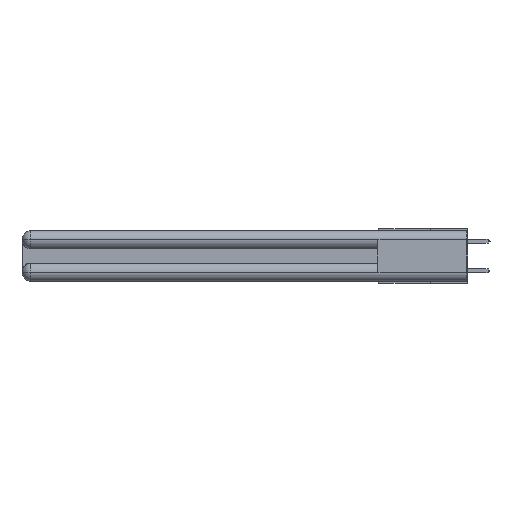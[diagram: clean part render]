
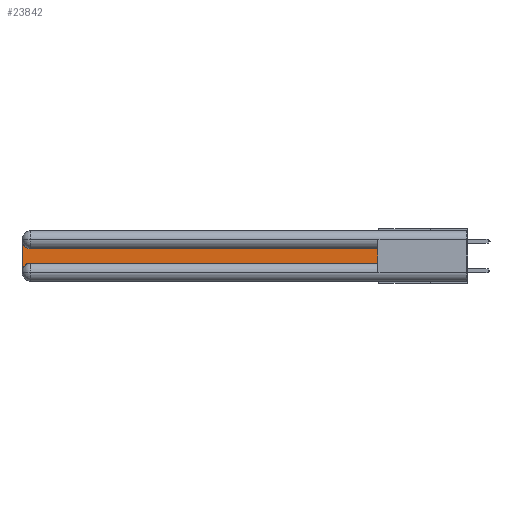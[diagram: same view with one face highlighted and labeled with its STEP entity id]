
A CAD part, left-side view. The second image highlights one B-rep face of the part: STEP entity #23842.
In plain terms, the highlighted planar face has unit normal (-1, 0, 0).
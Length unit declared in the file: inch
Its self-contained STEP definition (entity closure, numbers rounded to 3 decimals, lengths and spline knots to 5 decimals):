
#842 = VECTOR ( 'NONE', #8367, 39.37008 ) ;
#1450 = DIRECTION ( 'NONE',  ( 0., 0., -1. ) ) ;
#1662 = LINE ( 'NONE', #5142, #842 ) ;
#2708 = CARTESIAN_POINT ( 'NONE',  ( 0.075, 2.94, -0.0625 ) ) ;
#3270 = EDGE_LOOP ( 'NONE', ( #16878, #24091, #18093, #30044, #33054, #24185 ) ) ;
#4112 = LINE ( 'NONE', #25496, #29619 ) ;
#4541 = EDGE_CURVE ( 'NONE', #10692, #20927, #1662, .T. ) ;
#4879 = DIRECTION ( 'NONE',  ( 0., 0., -1. ) ) ;
#5142 = CARTESIAN_POINT ( 'NONE',  ( 0.075, 0.6, -0.2175 ) ) ;
#5673 = CIRCLE ( 'NONE', #33598, 0.06 ) ;
#5762 = VERTEX_POINT ( 'NONE', #7561 ) ;
#6572 = CARTESIAN_POINT ( 'NONE',  ( 0.075, 3., -0.0625 ) ) ;
#7421 = VECTOR ( 'NONE', #13288, 39.37008 ) ;
#7478 = EDGE_CURVE ( 'NONE', #5762, #22358, #5673, .T. ) ;
#7561 = CARTESIAN_POINT ( 'NONE',  ( 0.075, 2.94, -0.1225 ) ) ;
#8182 = DIRECTION ( 'NONE',  ( 0., 0., -1. ) ) ;
#8367 = DIRECTION ( 'NONE',  ( 0., -1., 0. ) ) ;
#8682 = AXIS2_PLACEMENT_3D ( 'NONE', #34301, #9982, #31364 ) ;
#9982 = DIRECTION ( 'NONE',  ( 1., 0., 0. ) ) ;
#10347 = CARTESIAN_POINT ( 'NONE',  ( 0.075, 0.6, -0.2175 ) ) ;
#10692 = VERTEX_POINT ( 'NONE', #21919 ) ;
#11008 = LINE ( 'NONE', #13211, #27294 ) ;
#11866 = FACE_OUTER_BOUND ( 'NONE', #3270, .T. ) ;
#12384 = CARTESIAN_POINT ( 'NONE',  ( 0.075, 3., -0.2775 ) ) ;
#12476 = CARTESIAN_POINT ( 'NONE',  ( 0.075, 3., -0.1225 ) ) ;
#13105 = VERTEX_POINT ( 'NONE', #28827 ) ;
#13211 = CARTESIAN_POINT ( 'NONE',  ( 0.075, 0.6, -0.1225 ) ) ;
#13288 = DIRECTION ( 'NONE',  ( 0., 0., 1. ) ) ;
#14334 = DIRECTION ( 'NONE',  ( 1., 0., 0. ) ) ;
#15075 = EDGE_CURVE ( 'NONE', #20927, #13105, #24165, .T. ) ;
#16878 = ORIENTED_EDGE ( 'NONE', *, *, #24099, .T. ) ;
#17084 = VERTEX_POINT ( 'NONE', #12384 ) ;
#18093 = ORIENTED_EDGE ( 'NONE', *, *, #25885, .T. ) ;
#20927 = VERTEX_POINT ( 'NONE', #22912 ) ;
#21372 = DIRECTION ( 'NONE',  ( 1., 0., 0. ) ) ;
#21919 = CARTESIAN_POINT ( 'NONE',  ( 0.075, 2.94, -0.2175 ) ) ;
#22358 = VERTEX_POINT ( 'NONE', #6572 ) ;
#22478 = AXIS2_PLACEMENT_3D ( 'NONE', #12476, #14334, #4879 ) ;
#22912 = CARTESIAN_POINT ( 'NONE',  ( 0.075, 0.6, -0.2175 ) ) ;
#23842 = ADVANCED_FACE ( 'NONE', ( #11866 ), #28568, .F. ) ;
#23926 = DIRECTION ( 'NONE',  ( 0., 1., 0. ) ) ;
#24091 = ORIENTED_EDGE ( 'NONE', *, *, #7478, .T. ) ;
#24099 = EDGE_CURVE ( 'NONE', #13105, #5762, #11008, .T. ) ;
#24165 = LINE ( 'NONE', #10347, #7421 ) ;
#24185 = ORIENTED_EDGE ( 'NONE', *, *, #15075, .T. ) ;
#25496 = CARTESIAN_POINT ( 'NONE',  ( 0.075, 3., -0.2175 ) ) ;
#25885 = EDGE_CURVE ( 'NONE', #22358, #17084, #4112, .T. ) ;
#27294 = VECTOR ( 'NONE', #23926, 39.37008 ) ;
#27766 = EDGE_CURVE ( 'NONE', #17084, #10692, #34576, .T. ) ;
#28568 = PLANE ( 'NONE',  #22478 ) ;
#28827 = CARTESIAN_POINT ( 'NONE',  ( 0.075, 0.6, -0.1225 ) ) ;
#29619 = VECTOR ( 'NONE', #1450, 39.37008 ) ;
#30044 = ORIENTED_EDGE ( 'NONE', *, *, #27766, .T. ) ;
#31364 = DIRECTION ( 'NONE',  ( 0., 0., -1. ) ) ;
#33054 = ORIENTED_EDGE ( 'NONE', *, *, #4541, .T. ) ;
#33598 = AXIS2_PLACEMENT_3D ( 'NONE', #2708, #21372, #8182 ) ;
#34301 = CARTESIAN_POINT ( 'NONE',  ( 0.075, 2.94, -0.2775 ) ) ;
#34576 = CIRCLE ( 'NONE', #8682, 0.06 ) ;
